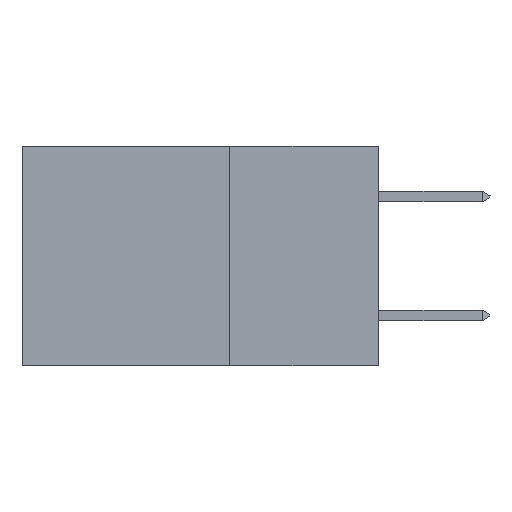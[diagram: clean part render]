
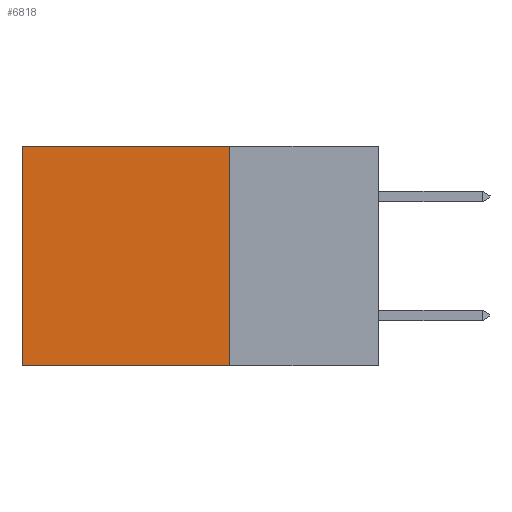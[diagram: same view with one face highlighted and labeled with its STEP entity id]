
A CAD part, left-side view. The second image highlights one B-rep face of the part: STEP entity #6818.
In plain terms, the highlighted planar face has unit normal (-1, 0, 0).
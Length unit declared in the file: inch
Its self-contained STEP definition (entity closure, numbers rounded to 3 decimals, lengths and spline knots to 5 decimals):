
#674 = LINE ( 'NONE', #7987, #21301 ) ;
#968 = EDGE_CURVE ( 'NONE', #16876, #17180, #14328, .T. ) ;
#3784 = DIRECTION ( 'NONE',  ( 0., 0., -1. ) ) ;
#5006 = DIRECTION ( 'NONE',  ( 0., 0., -1. ) ) ;
#5708 = CARTESIAN_POINT ( 'NONE',  ( 0.2615, 0.25, -0.37 ) ) ;
#5850 = VERTEX_POINT ( 'NONE', #12825 ) ;
#6818 = ADVANCED_FACE ( 'NONE', ( #21704 ), #19773, .F. ) ;
#7038 = EDGE_CURVE ( 'NONE', #20291, #5850, #7626, .T. ) ;
#7154 = CARTESIAN_POINT ( 'NONE',  ( 0.2615, 0.25, -0.37 ) ) ;
#7626 = LINE ( 'NONE', #16646, #8104 ) ;
#7668 = VECTOR ( 'NONE', #17701, 39.37008 ) ;
#7987 = CARTESIAN_POINT ( 'NONE',  ( 0.2615, 0.25, -0.37 ) ) ;
#8104 = VECTOR ( 'NONE', #3784, 39.37008 ) ;
#8117 = CARTESIAN_POINT ( 'NONE',  ( 0.2615, 0.25, 0. ) ) ;
#9197 = AXIS2_PLACEMENT_3D ( 'NONE', #7154, #21818, #5006 ) ;
#10336 = ORIENTED_EDGE ( 'NONE', *, *, #7038, .T. ) ;
#12087 = CARTESIAN_POINT ( 'NONE',  ( 0.2615, 0.6, 0. ) ) ;
#12825 = CARTESIAN_POINT ( 'NONE',  ( 0.2615, 0.6, -0.37 ) ) ;
#12890 = CARTESIAN_POINT ( 'NONE',  ( 0.2615, 0.25, 0. ) ) ;
#13188 = ORIENTED_EDGE ( 'NONE', *, *, #13232, .F. ) ;
#13232 = EDGE_CURVE ( 'NONE', #17180, #5850, #674, .T. ) ;
#13551 = DIRECTION ( 'NONE',  ( 0., 1., 0. ) ) ;
#13773 = DIRECTION ( 'NONE',  ( 0., 1., 0. ) ) ;
#14235 = EDGE_LOOP ( 'NONE', ( #10336, #13188, #14790, #16696 ) ) ;
#14328 = LINE ( 'NONE', #21663, #7668 ) ;
#14790 = ORIENTED_EDGE ( 'NONE', *, *, #968, .F. ) ;
#16646 = CARTESIAN_POINT ( 'NONE',  ( 0.2615, 0.6, -0.37 ) ) ;
#16696 = ORIENTED_EDGE ( 'NONE', *, *, #17616, .T. ) ;
#16876 = VERTEX_POINT ( 'NONE', #12890 ) ;
#17180 = VERTEX_POINT ( 'NONE', #5708 ) ;
#17616 = EDGE_CURVE ( 'NONE', #16876, #20291, #20750, .T. ) ;
#17701 = DIRECTION ( 'NONE',  ( 0., 0., -1. ) ) ;
#19773 = PLANE ( 'NONE',  #9197 ) ;
#20291 = VERTEX_POINT ( 'NONE', #12087 ) ;
#20750 = LINE ( 'NONE', #8117, #23129 ) ;
#21301 = VECTOR ( 'NONE', #13773, 39.37008 ) ;
#21663 = CARTESIAN_POINT ( 'NONE',  ( 0.2615, 0.25, -0.37 ) ) ;
#21704 = FACE_OUTER_BOUND ( 'NONE', #14235, .T. ) ;
#21818 = DIRECTION ( 'NONE',  ( 1., 0., 0. ) ) ;
#23129 = VECTOR ( 'NONE', #13551, 39.37008 ) ;
